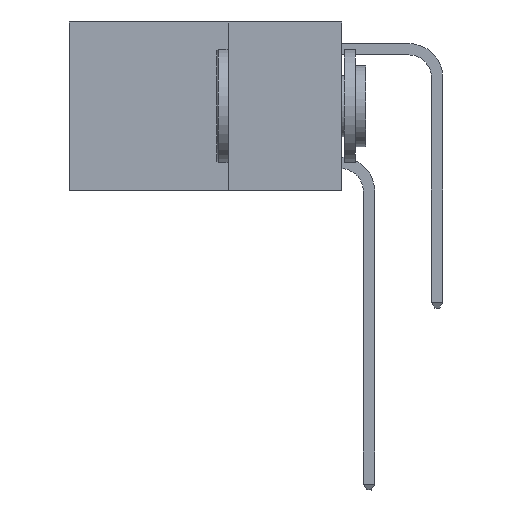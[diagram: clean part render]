
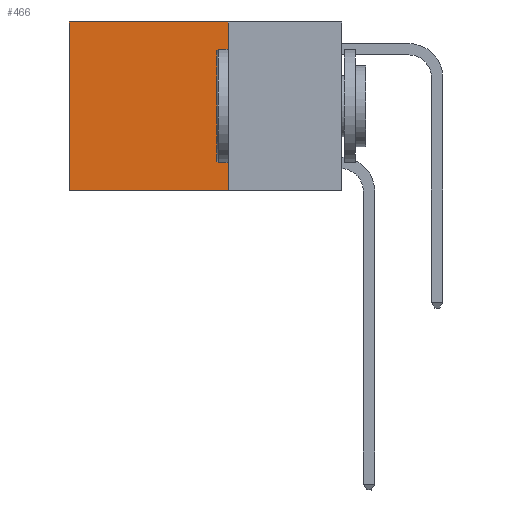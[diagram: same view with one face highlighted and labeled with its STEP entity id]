
A CAD part, left-side view. The second image highlights one B-rep face of the part: STEP entity #466.
In plain terms, the highlighted planar face has unit normal (-1, 0, 0).
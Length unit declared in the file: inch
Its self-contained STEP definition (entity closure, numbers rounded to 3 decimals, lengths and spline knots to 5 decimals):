
#251 = VECTOR ( 'NONE', #12916, 39.37008 ) ;
#322 = AXIS2_PLACEMENT_3D ( 'NONE', #14649, #2509, #5312 ) ;
#466 = ADVANCED_FACE ( 'NONE', ( #14364 ), #5647, .F. ) ;
#781 = ORIENTED_EDGE ( 'NONE', *, *, #11055, .F. ) ;
#1854 = ORIENTED_EDGE ( 'NONE', *, *, #8179, .T. ) ;
#2354 = ORIENTED_EDGE ( 'NONE', *, *, #8752, .T. ) ;
#2509 = DIRECTION ( 'NONE',  ( 1., 0., 0. ) ) ;
#2760 = VERTEX_POINT ( 'NONE', #11720 ) ;
#3782 = VERTEX_POINT ( 'NONE', #12977 ) ;
#3816 = LINE ( 'NONE', #5888, #12171 ) ;
#4599 = LINE ( 'NONE', #11375, #10685 ) ;
#4935 = CARTESIAN_POINT ( 'NONE',  ( 0.2625, 0.25, 0. ) ) ;
#5312 = DIRECTION ( 'NONE',  ( 0., 0., -1. ) ) ;
#5647 = PLANE ( 'NONE',  #322 ) ;
#5888 = CARTESIAN_POINT ( 'NONE',  ( 0.2625, 0.25, -0.37 ) ) ;
#5907 = CARTESIAN_POINT ( 'NONE',  ( 0.2625, 0.25, 0. ) ) ;
#6410 = LINE ( 'NONE', #4935, #251 ) ;
#8140 = LINE ( 'NONE', #5907, #8500 ) ;
#8179 = EDGE_CURVE ( 'NONE', #11470, #3782, #8140, .T. ) ;
#8491 = EDGE_LOOP ( 'NONE', ( #2354, #10999, #781, #1854 ) ) ;
#8500 = VECTOR ( 'NONE', #13863, 39.37008 ) ;
#8752 = EDGE_CURVE ( 'NONE', #3782, #13000, #4599, .T. ) ;
#10389 = EDGE_CURVE ( 'NONE', #2760, #13000, #3816, .T. ) ;
#10685 = VECTOR ( 'NONE', #12497, 39.37008 ) ;
#10999 = ORIENTED_EDGE ( 'NONE', *, *, #10389, .F. ) ;
#11055 = EDGE_CURVE ( 'NONE', #11470, #2760, #6410, .T. ) ;
#11334 = CARTESIAN_POINT ( 'NONE',  ( 0.2625, 0.25, 0. ) ) ;
#11375 = CARTESIAN_POINT ( 'NONE',  ( 0.2625, 0.6, 0. ) ) ;
#11470 = VERTEX_POINT ( 'NONE', #11334 ) ;
#11720 = CARTESIAN_POINT ( 'NONE',  ( 0.2625, 0.25, -0.37 ) ) ;
#12171 = VECTOR ( 'NONE', #13847, 39.37008 ) ;
#12497 = DIRECTION ( 'NONE',  ( 0., 0., -1. ) ) ;
#12916 = DIRECTION ( 'NONE',  ( 0., 0., -1. ) ) ;
#12977 = CARTESIAN_POINT ( 'NONE',  ( 0.2625, 0.6, 0. ) ) ;
#13000 = VERTEX_POINT ( 'NONE', #13643 ) ;
#13643 = CARTESIAN_POINT ( 'NONE',  ( 0.2625, 0.6, -0.37 ) ) ;
#13847 = DIRECTION ( 'NONE',  ( 0., 1., 0. ) ) ;
#13863 = DIRECTION ( 'NONE',  ( 0., 1., 0. ) ) ;
#14364 = FACE_OUTER_BOUND ( 'NONE', #8491, .T. ) ;
#14649 = CARTESIAN_POINT ( 'NONE',  ( 0.2625, 0.25, 0. ) ) ;
